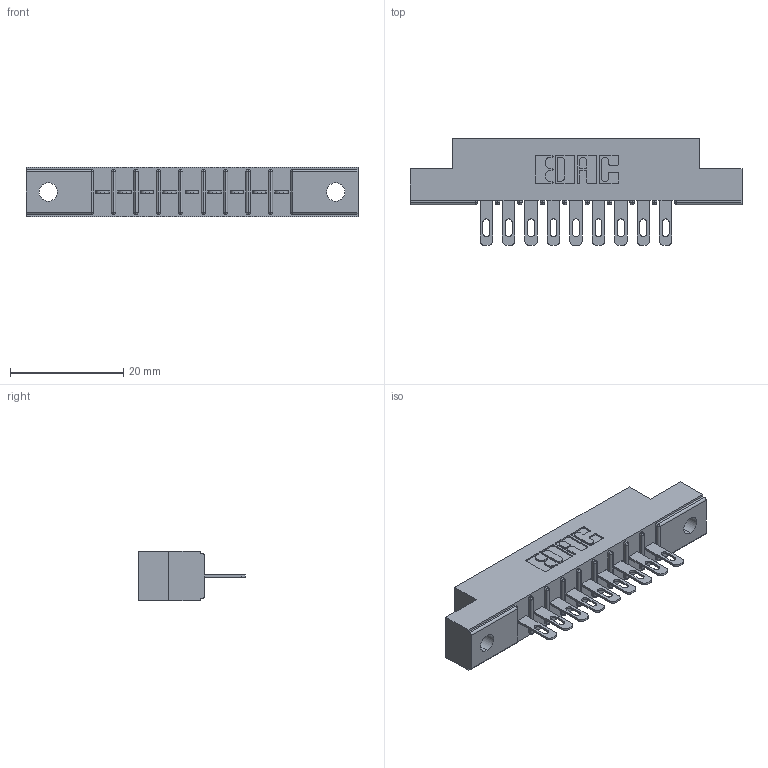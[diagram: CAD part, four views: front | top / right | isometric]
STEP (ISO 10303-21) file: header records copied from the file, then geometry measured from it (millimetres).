
FILE_DESCRIPTION (( 'STEP AP203' ), '1' );
FILE_NAME ('356-009-400-102.STEP', '2020-09-23T09:24:39', ( '' ), ( '' ), 'SwSTEP 2.0', 'SolidWorks 2020', '' );
FILE_SCHEMA (( 'CONFIG_CONTROL_DESIGN' ));
Length unit declared in the file: inch
Products named in the file (3): 306-290-001_100; 306 Part_.128 Dia; 356-009-400-102
Assembly tree (10 placements, depth 2):
  356-009-400-102
    306 Part_.128 Dia
    306-290-001_100  x9
Bounding box: 58.67 x 18.87 x 8.71 mm (x, y, z)
Volume: 3943.8 mm3; surface area: 5312.4 mm2
Topology: 10 solids, 10 shells, 800 faces, 2251 edges, 1450 vertices
Faces by surface type: plane 518, cylinder 246, sphere 36
Entity records: 12834 total; most frequent: CARTESIAN_POINT 2150, ORIENTED_EDGE 2126, DIRECTION 2125, EDGE_CURVE 1063, VECTOR 811, LINE 811, VERTEX_POINT 682, AXIS2_PLACEMENT_3D 657
